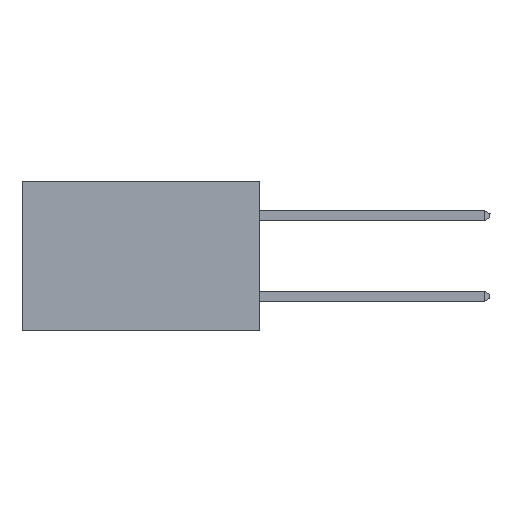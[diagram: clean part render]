
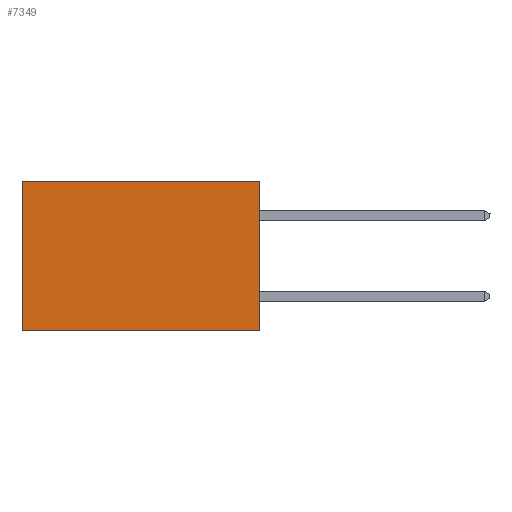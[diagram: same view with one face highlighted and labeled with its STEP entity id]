
A CAD part, left-side view. The second image highlights one B-rep face of the part: STEP entity #7349.
In plain terms, the highlighted planar face has unit normal (-1, 0, 0).
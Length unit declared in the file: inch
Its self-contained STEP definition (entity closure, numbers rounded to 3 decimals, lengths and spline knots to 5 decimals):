
#280 = AXIS2_PLACEMENT_3D ( 'NONE', #10465, #11573, #4979 ) ;
#422 = CARTESIAN_POINT ( 'NONE',  ( 0.277, 0., -0.37 ) ) ;
#703 = DIRECTION ( 'NONE',  ( 0., 1., 0. ) ) ;
#852 = LINE ( 'NONE', #422, #9780 ) ;
#1375 = EDGE_CURVE ( 'NONE', #6402, #7818, #852, .T. ) ;
#1405 = EDGE_CURVE ( 'NONE', #12464, #6402, #6157, .T. ) ;
#1747 = ORIENTED_EDGE ( 'NONE', *, *, #14142, .T. ) ;
#2124 = DIRECTION ( 'NONE',  ( 0., 1., 0. ) ) ;
#2494 = PLANE ( 'NONE',  #280 ) ;
#2528 = CARTESIAN_POINT ( 'NONE',  ( 0.277, 0.59, 0. ) ) ;
#2821 = CARTESIAN_POINT ( 'NONE',  ( 0.277, 0., 0. ) ) ;
#3029 = VECTOR ( 'NONE', #5359, 39.37008 ) ;
#3851 = EDGE_CURVE ( 'NONE', #12464, #13266, #9146, .T. ) ;
#4418 = CARTESIAN_POINT ( 'NONE',  ( 0.277, 0.59, -0.37 ) ) ;
#4640 = CARTESIAN_POINT ( 'NONE',  ( 0.277, 0., 0. ) ) ;
#4888 = CARTESIAN_POINT ( 'NONE',  ( 0.277, 0., -0.37 ) ) ;
#4979 = DIRECTION ( 'NONE',  ( 0., 0., -1. ) ) ;
#5338 = ORIENTED_EDGE ( 'NONE', *, *, #3851, .T. ) ;
#5359 = DIRECTION ( 'NONE',  ( 0., 0., -1. ) ) ;
#6157 = LINE ( 'NONE', #9815, #3029 ) ;
#6240 = EDGE_LOOP ( 'NONE', ( #1747, #10626, #13529, #5338 ) ) ;
#6402 = VERTEX_POINT ( 'NONE', #4888 ) ;
#7349 = ADVANCED_FACE ( 'NONE', ( #11986 ), #2494, .F. ) ;
#7553 = VECTOR ( 'NONE', #11454, 39.37008 ) ;
#7818 = VERTEX_POINT ( 'NONE', #4418 ) ;
#9146 = LINE ( 'NONE', #4640, #12089 ) ;
#9780 = VECTOR ( 'NONE', #703, 39.37008 ) ;
#9815 = CARTESIAN_POINT ( 'NONE',  ( 0.277, 0., -0.37 ) ) ;
#10344 = CARTESIAN_POINT ( 'NONE',  ( 0.277, 0.59, -0.37 ) ) ;
#10465 = CARTESIAN_POINT ( 'NONE',  ( 0.277, 0., -0.37 ) ) ;
#10626 = ORIENTED_EDGE ( 'NONE', *, *, #1375, .F. ) ;
#10871 = LINE ( 'NONE', #10344, #7553 ) ;
#11454 = DIRECTION ( 'NONE',  ( 0., 0., -1. ) ) ;
#11573 = DIRECTION ( 'NONE',  ( 1., 0., 0. ) ) ;
#11986 = FACE_OUTER_BOUND ( 'NONE', #6240, .T. ) ;
#12089 = VECTOR ( 'NONE', #2124, 39.37008 ) ;
#12464 = VERTEX_POINT ( 'NONE', #2821 ) ;
#13266 = VERTEX_POINT ( 'NONE', #2528 ) ;
#13529 = ORIENTED_EDGE ( 'NONE', *, *, #1405, .F. ) ;
#14142 = EDGE_CURVE ( 'NONE', #13266, #7818, #10871, .T. ) ;
